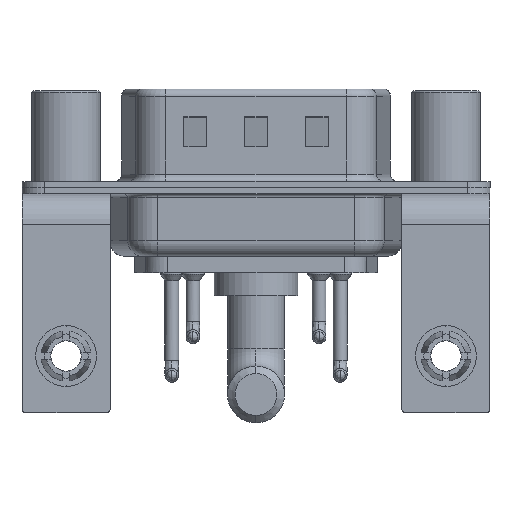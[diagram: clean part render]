
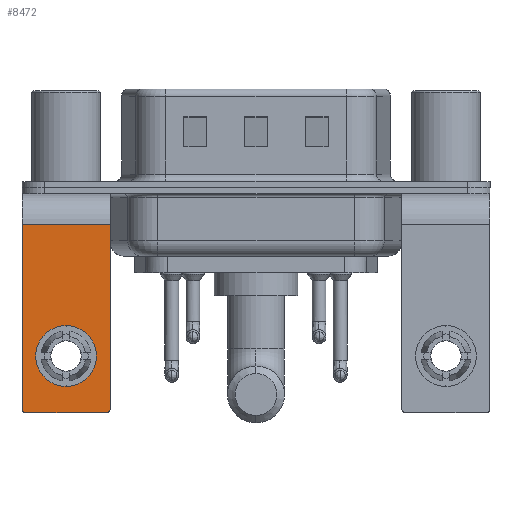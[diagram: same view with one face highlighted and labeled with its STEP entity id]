
A CAD part, front view. The second image highlights one B-rep face of the part: STEP entity #8472.
In plain terms, the highlighted planar face has unit normal (0, -1, 0).
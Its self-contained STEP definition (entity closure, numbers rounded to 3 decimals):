
#49 = EDGE_CURVE ( 'NONE', #22401, #2997, #10184, .T. ) ;
#222 = ORIENTED_EDGE ( 'NONE', *, *, #49, .F. ) ;
#779 = CARTESIAN_POINT ( 'NONE',  ( 2.65, -6.25, -14.55 ) ) ;
#843 = CARTESIAN_POINT ( 'NONE',  ( 0., -6.25, -13.07 ) ) ;
#886 = DIRECTION ( 'NONE',  ( 0., 0., 1. ) ) ;
#1066 = CARTESIAN_POINT ( 'NONE',  ( 2.9, -6.25, -14.55 ) ) ;
#1461 = DIRECTION ( 'NONE',  ( 0., 1., 0. ) ) ;
#1634 = CARTESIAN_POINT ( 'NONE',  ( -2.9, -6.25, -2.4 ) ) ;
#2228 = CIRCLE ( 'NONE', #12940, 0.25 ) ;
#2371 = VERTEX_POINT ( 'NONE', #16010 ) ;
#2512 = VECTOR ( 'NONE', #4992, 1000. ) ;
#2801 = FACE_OUTER_BOUND ( 'NONE', #15784, .T. ) ;
#2997 = VERTEX_POINT ( 'NONE', #14365 ) ;
#3364 = CARTESIAN_POINT ( 'NONE',  ( -2.9, -6.25, -2.4 ) ) ;
#3396 = CARTESIAN_POINT ( 'NONE',  ( -2.65, -6.25, -14.55 ) ) ;
#3518 = CARTESIAN_POINT ( 'NONE',  ( 2.65, -6.25, -14.8 ) ) ;
#4404 = DIRECTION ( 'NONE',  ( -1., 0., 0. ) ) ;
#4474 = DIRECTION ( 'NONE',  ( 0., -1., 0. ) ) ;
#4977 = EDGE_LOOP ( 'NONE', ( #5423, #17395 ) ) ;
#4992 = DIRECTION ( 'NONE',  ( 0., 0., -1. ) ) ;
#5158 = AXIS2_PLACEMENT_3D ( 'NONE', #17746, #1461, #10492 ) ;
#5423 = ORIENTED_EDGE ( 'NONE', *, *, #10115, .T. ) ;
#5493 = ORIENTED_EDGE ( 'NONE', *, *, #7192, .F. ) ;
#6526 = VERTEX_POINT ( 'NONE', #1066 ) ;
#7192 = EDGE_CURVE ( 'NONE', #9432, #6526, #18918, .T. ) ;
#7325 = DIRECTION ( 'NONE',  ( 0., -1., 0. ) ) ;
#7529 = DIRECTION ( 'NONE',  ( 0., 1., 0. ) ) ;
#7958 = CARTESIAN_POINT ( 'NONE',  ( 2.9, -6.25, -2.4 ) ) ;
#8140 = PLANE ( 'NONE',  #13964 ) ;
#8472 = ADVANCED_FACE ( 'NONE', ( #17249, #2801 ), #8140, .F. ) ;
#9197 = VERTEX_POINT ( 'NONE', #3364 ) ;
#9432 = VERTEX_POINT ( 'NONE', #7958 ) ;
#9878 = CARTESIAN_POINT ( 'NONE',  ( 0., -6.25, -9.07 ) ) ;
#10115 = EDGE_CURVE ( 'NONE', #13063, #19704, #22512, .T. ) ;
#10184 = LINE ( 'NONE', #15697, #13184 ) ;
#10249 = DIRECTION ( 'NONE',  ( 0., 0., -1. ) ) ;
#10492 = DIRECTION ( 'NONE',  ( 0., 0., 1. ) ) ;
#10657 = VECTOR ( 'NONE', #10249, 1000. ) ;
#11234 = CARTESIAN_POINT ( 'NONE',  ( 0., -6.25, -11.07 ) ) ;
#11506 = ORIENTED_EDGE ( 'NONE', *, *, #17708, .T. ) ;
#11764 = VECTOR ( 'NONE', #4404, 1000. ) ;
#12043 = LINE ( 'NONE', #1634, #2512 ) ;
#12940 = AXIS2_PLACEMENT_3D ( 'NONE', #3396, #7325, #14353 ) ;
#13063 = VERTEX_POINT ( 'NONE', #843 ) ;
#13183 = CARTESIAN_POINT ( 'NONE',  ( 2.9, -6.25, -2.4 ) ) ;
#13184 = VECTOR ( 'NONE', #18965, 1000. ) ;
#13681 = DIRECTION ( 'NONE',  ( 0., 1., 0. ) ) ;
#13964 = AXIS2_PLACEMENT_3D ( 'NONE', #20959, #13681, #22705 ) ;
#14353 = DIRECTION ( 'NONE',  ( 0., 0., 1. ) ) ;
#14365 = CARTESIAN_POINT ( 'NONE',  ( -2.65, -6.25, -14.8 ) ) ;
#14423 = ORIENTED_EDGE ( 'NONE', *, *, #20409, .T. ) ;
#14448 = AXIS2_PLACEMENT_3D ( 'NONE', #779, #4474, #886 ) ;
#15697 = CARTESIAN_POINT ( 'NONE',  ( 2.9, -6.25, -14.8 ) ) ;
#15784 = EDGE_LOOP ( 'NONE', ( #20022, #11506, #222, #14423, #5493, #16278 ) ) ;
#15888 = EDGE_CURVE ( 'NONE', #9432, #9197, #22102, .T. ) ;
#16010 = CARTESIAN_POINT ( 'NONE',  ( -2.9, -6.25, -14.55 ) ) ;
#16019 = EDGE_CURVE ( 'NONE', #9197, #2371, #12043, .T. ) ;
#16278 = ORIENTED_EDGE ( 'NONE', *, *, #15888, .T. ) ;
#17249 = FACE_BOUND ( 'NONE', #4977, .T. ) ;
#17395 = ORIENTED_EDGE ( 'NONE', *, *, #22854, .T. ) ;
#17708 = EDGE_CURVE ( 'NONE', #2371, #2997, #2228, .T. ) ;
#17746 = CARTESIAN_POINT ( 'NONE',  ( 0., -6.25, -11.07 ) ) ;
#18918 = LINE ( 'NONE', #22504, #10657 ) ;
#18965 = DIRECTION ( 'NONE',  ( -1., 0., 0. ) ) ;
#18985 = CIRCLE ( 'NONE', #20835, 2. ) ;
#19704 = VERTEX_POINT ( 'NONE', #9878 ) ;
#20022 = ORIENTED_EDGE ( 'NONE', *, *, #16019, .T. ) ;
#20409 = EDGE_CURVE ( 'NONE', #22401, #6526, #22593, .T. ) ;
#20835 = AXIS2_PLACEMENT_3D ( 'NONE', #11234, #7529, #21623 ) ;
#20959 = CARTESIAN_POINT ( 'NONE',  ( 2.9, -6.25, -2.4 ) ) ;
#21623 = DIRECTION ( 'NONE',  ( 0., 0., 1. ) ) ;
#22102 = LINE ( 'NONE', #13183, #11764 ) ;
#22401 = VERTEX_POINT ( 'NONE', #3518 ) ;
#22504 = CARTESIAN_POINT ( 'NONE',  ( 2.9, -6.25, -2.4 ) ) ;
#22512 = CIRCLE ( 'NONE', #5158, 2. ) ;
#22593 = CIRCLE ( 'NONE', #14448, 0.25 ) ;
#22705 = DIRECTION ( 'NONE',  ( 0., 0., 1. ) ) ;
#22854 = EDGE_CURVE ( 'NONE', #19704, #13063, #18985, .T. ) ;
